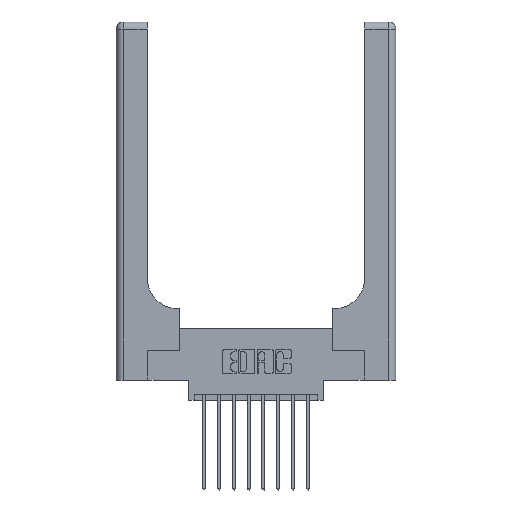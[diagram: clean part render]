
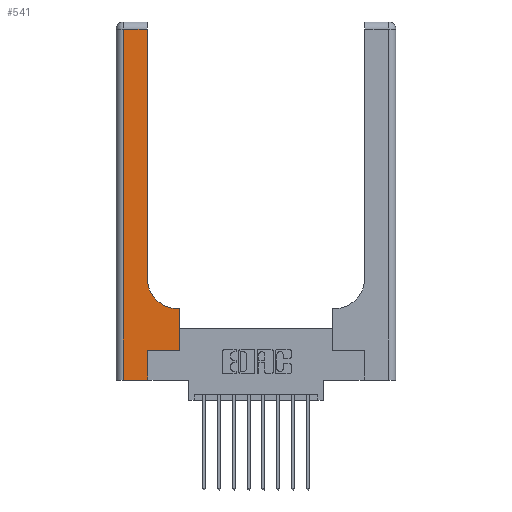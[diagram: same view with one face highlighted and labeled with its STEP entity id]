
A CAD part, top view. The second image highlights one B-rep face of the part: STEP entity #541.
In plain terms, the highlighted planar face has unit normal (0, 0, 1).
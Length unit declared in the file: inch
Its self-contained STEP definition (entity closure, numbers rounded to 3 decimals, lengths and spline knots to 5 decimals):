
#264 = ORIENTED_EDGE ( 'NONE', *, *, #11575, .T. ) ;
#541 = ADVANCED_FACE ( 'NONE', ( #12513 ), #13294, .F. ) ;
#918 = VECTOR ( 'NONE', #14700, 39.37008 ) ;
#1049 = DIRECTION ( 'NONE',  ( -1., 0., 0. ) ) ;
#1052 = LINE ( 'NONE', #8599, #8020 ) ;
#1118 = VERTEX_POINT ( 'NONE', #10555 ) ;
#1122 = LINE ( 'NONE', #9692, #13192 ) ;
#1229 = DIRECTION ( 'NONE',  ( 0., 0., -1. ) ) ;
#1522 = DIRECTION ( 'NONE',  ( 0., 1., 0. ) ) ;
#1663 = CARTESIAN_POINT ( 'NONE',  ( 0.528, 0.6, 0.37 ) ) ;
#1717 = VERTEX_POINT ( 'NONE', #1663 ) ;
#1914 = VERTEX_POINT ( 'NONE', #2167 ) ;
#1915 = CARTESIAN_POINT ( 'NONE',  ( 0.06, 2.94, 0.37 ) ) ;
#2014 = EDGE_CURVE ( 'NONE', #1118, #8633, #13185, .T. ) ;
#2128 = ORIENTED_EDGE ( 'NONE', *, *, #11601, .T. ) ;
#2167 = CARTESIAN_POINT ( 'NONE',  ( 0.06, 0., 0.37 ) ) ;
#2619 = EDGE_CURVE ( 'NONE', #8474, #11223, #14792, .T. ) ;
#2762 = VECTOR ( 'NONE', #7060, 39.37008 ) ;
#3185 = CARTESIAN_POINT ( 'NONE',  ( 0.26, 0.85, 0.37 ) ) ;
#3248 = VECTOR ( 'NONE', #8819, 39.37008 ) ;
#3678 = DIRECTION ( 'NONE',  ( 1., 0., 0. ) ) ;
#4112 = VECTOR ( 'NONE', #1049, 39.37008 ) ;
#4263 = CARTESIAN_POINT ( 'NONE',  ( 0.26, 2.94, 0.37 ) ) ;
#4971 = VERTEX_POINT ( 'NONE', #4263 ) ;
#5290 = CARTESIAN_POINT ( 'NONE',  ( 0.26, 3., 0.37 ) ) ;
#5328 = DIRECTION ( 'NONE',  ( 0., 0., -1. ) ) ;
#5440 = VECTOR ( 'NONE', #1522, 39.37008 ) ;
#6549 = EDGE_LOOP ( 'NONE', ( #8157, #8528, #9253, #264, #13444, #7625, #2128, #11829, #10422 ) ) ;
#7060 = DIRECTION ( 'NONE',  ( 0., 1., 0. ) ) ;
#7625 = ORIENTED_EDGE ( 'NONE', *, *, #7758, .T. ) ;
#7758 = EDGE_CURVE ( 'NONE', #11223, #9214, #1122, .T. ) ;
#7967 = EDGE_CURVE ( 'NONE', #4971, #7987, #10264, .T. ) ;
#7987 = VERTEX_POINT ( 'NONE', #1915 ) ;
#8020 = VECTOR ( 'NONE', #14445, 39.37008 ) ;
#8069 = CARTESIAN_POINT ( 'NONE',  ( 0.26, 0.6, 0.37 ) ) ;
#8157 = ORIENTED_EDGE ( 'NONE', *, *, #11778, .T. ) ;
#8246 = CARTESIAN_POINT ( 'NONE',  ( 0.51, 0.85, 0.37 ) ) ;
#8474 = VERTEX_POINT ( 'NONE', #8794 ) ;
#8522 = CARTESIAN_POINT ( 'NONE',  ( 0.528, 0.25, 0.37 ) ) ;
#8528 = ORIENTED_EDGE ( 'NONE', *, *, #7967, .T. ) ;
#8599 = CARTESIAN_POINT ( 'NONE',  ( 0.06, 3., 0.37 ) ) ;
#8633 = VERTEX_POINT ( 'NONE', #3185 ) ;
#8794 = CARTESIAN_POINT ( 'NONE',  ( 0.265, 0., 0.37 ) ) ;
#8819 = DIRECTION ( 'NONE',  ( 0., 1., 0. ) ) ;
#9195 = DIRECTION ( 'NONE',  ( -1., 0., 0. ) ) ;
#9214 = VERTEX_POINT ( 'NONE', #12790 ) ;
#9253 = ORIENTED_EDGE ( 'NONE', *, *, #11021, .T. ) ;
#9426 = DIRECTION ( 'NONE',  ( 1., 0., 0. ) ) ;
#9461 = LINE ( 'NONE', #5290, #3248 ) ;
#9494 = CARTESIAN_POINT ( 'NONE',  ( 0., 3., 0.37 ) ) ;
#9692 = CARTESIAN_POINT ( 'NONE',  ( 0.265, 0.25, 0.37 ) ) ;
#10264 = LINE ( 'NONE', #13546, #918 ) ;
#10307 = LINE ( 'NONE', #8069, #4112 ) ;
#10422 = ORIENTED_EDGE ( 'NONE', *, *, #2014, .T. ) ;
#10555 = CARTESIAN_POINT ( 'NONE',  ( 0.51, 0.6, 0.37 ) ) ;
#10712 = CARTESIAN_POINT ( 'NONE',  ( 0., 0., 0.37 ) ) ;
#11021 = EDGE_CURVE ( 'NONE', #7987, #1914, #1052, .T. ) ;
#11223 = VERTEX_POINT ( 'NONE', #11252 ) ;
#11252 = CARTESIAN_POINT ( 'NONE',  ( 0.265, 0.25, 0.37 ) ) ;
#11378 = AXIS2_PLACEMENT_3D ( 'NONE', #9494, #5328, #9195 ) ;
#11575 = EDGE_CURVE ( 'NONE', #1914, #8474, #12399, .T. ) ;
#11601 = EDGE_CURVE ( 'NONE', #9214, #1717, #14382, .T. ) ;
#11778 = EDGE_CURVE ( 'NONE', #8633, #4971, #9461, .T. ) ;
#11829 = ORIENTED_EDGE ( 'NONE', *, *, #14305, .T. ) ;
#12399 = LINE ( 'NONE', #10712, #15094 ) ;
#12513 = FACE_OUTER_BOUND ( 'NONE', #6549, .T. ) ;
#12790 = CARTESIAN_POINT ( 'NONE',  ( 0.528, 0.25, 0.37 ) ) ;
#12866 = CARTESIAN_POINT ( 'NONE',  ( 0.265, 0., 0.37 ) ) ;
#13185 = CIRCLE ( 'NONE', #14872, 0.25 ) ;
#13192 = VECTOR ( 'NONE', #14366, 39.37008 ) ;
#13294 = PLANE ( 'NONE',  #11378 ) ;
#13444 = ORIENTED_EDGE ( 'NONE', *, *, #2619, .T. ) ;
#13546 = CARTESIAN_POINT ( 'NONE',  ( 0., 2.94, 0.37 ) ) ;
#14305 = EDGE_CURVE ( 'NONE', #1717, #1118, #10307, .T. ) ;
#14366 = DIRECTION ( 'NONE',  ( 1., 0., 0. ) ) ;
#14382 = LINE ( 'NONE', #8522, #5440 ) ;
#14445 = DIRECTION ( 'NONE',  ( 0., -1., 0. ) ) ;
#14700 = DIRECTION ( 'NONE',  ( -1., 0., 0. ) ) ;
#14792 = LINE ( 'NONE', #12866, #2762 ) ;
#14872 = AXIS2_PLACEMENT_3D ( 'NONE', #8246, #1229, #9426 ) ;
#15094 = VECTOR ( 'NONE', #3678, 39.37008 ) ;
